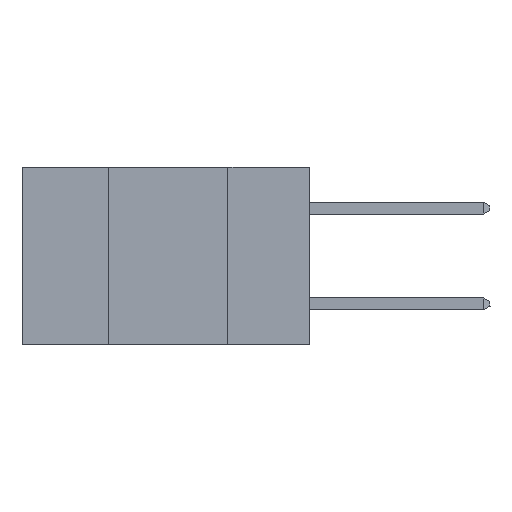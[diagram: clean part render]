
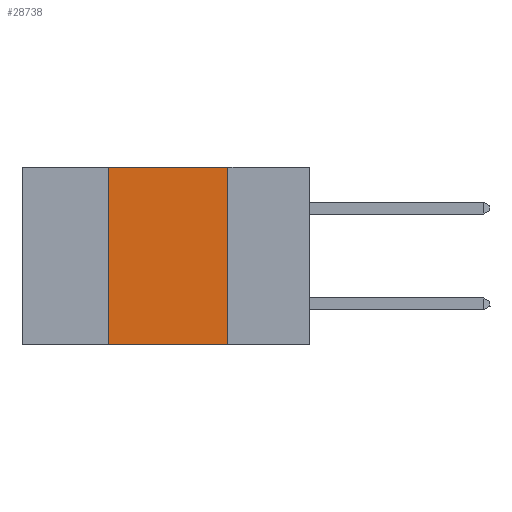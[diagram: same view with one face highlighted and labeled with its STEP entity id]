
A CAD part, left-side view. The second image highlights one B-rep face of the part: STEP entity #28738.
In plain terms, the highlighted planar face has unit normal (-1, 0, 0).
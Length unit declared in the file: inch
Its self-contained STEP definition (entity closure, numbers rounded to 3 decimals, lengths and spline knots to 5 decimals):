
#264 = PLANE ( 'NONE',  #30064 ) ;
#455 = CARTESIAN_POINT ( 'NONE',  ( 0., 0.42, 0. ) ) ;
#532 = VERTEX_POINT ( 'NONE', #7471 ) ;
#3584 = ORIENTED_EDGE ( 'NONE', *, *, #12356, .T. ) ;
#3883 = VECTOR ( 'NONE', #11330, 39.37008 ) ;
#3884 = EDGE_CURVE ( 'NONE', #7763, #26362, #16132, .T. ) ;
#7471 = CARTESIAN_POINT ( 'NONE',  ( 0., 0.17, -0.37 ) ) ;
#7547 = VECTOR ( 'NONE', #19287, 39.37008 ) ;
#7763 = VERTEX_POINT ( 'NONE', #20365 ) ;
#9404 = VECTOR ( 'NONE', #25095, 39.37008 ) ;
#11330 = DIRECTION ( 'NONE',  ( 0., -1., 0. ) ) ;
#12356 = EDGE_CURVE ( 'NONE', #7763, #532, #16015, .T. ) ;
#13783 = VERTEX_POINT ( 'NONE', #23346 ) ;
#14371 = EDGE_CURVE ( 'NONE', #26362, #13783, #29298, .T. ) ;
#16015 = LINE ( 'NONE', #26833, #3883 ) ;
#16132 = LINE ( 'NONE', #455, #20914 ) ;
#16338 = EDGE_LOOP ( 'NONE', ( #22075, #16587, #23740, #3584 ) ) ;
#16587 = ORIENTED_EDGE ( 'NONE', *, *, #14371, .F. ) ;
#18638 = DIRECTION ( 'NONE',  ( 0., 0., 1. ) ) ;
#19287 = DIRECTION ( 'NONE',  ( 0., -1., 0. ) ) ;
#19853 = CARTESIAN_POINT ( 'NONE',  ( 0., 0.42, 0. ) ) ;
#20365 = CARTESIAN_POINT ( 'NONE',  ( 0., 0.42, -0.37 ) ) ;
#20914 = VECTOR ( 'NONE', #18638, 39.37008 ) ;
#22075 = ORIENTED_EDGE ( 'NONE', *, *, #31052, .F. ) ;
#22120 = CARTESIAN_POINT ( 'NONE',  ( 0., 0.17, 0. ) ) ;
#22927 = DIRECTION ( 'NONE',  ( 0., 0., -1. ) ) ;
#23346 = CARTESIAN_POINT ( 'NONE',  ( 0., 0.17, 0. ) ) ;
#23740 = ORIENTED_EDGE ( 'NONE', *, *, #3884, .F. ) ;
#25095 = DIRECTION ( 'NONE',  ( 0., 0., -1. ) ) ;
#25277 = DIRECTION ( 'NONE',  ( 1., 0., 0. ) ) ;
#26362 = VERTEX_POINT ( 'NONE', #19853 ) ;
#26481 = CARTESIAN_POINT ( 'NONE',  ( 0., 0.6, 0. ) ) ;
#26833 = CARTESIAN_POINT ( 'NONE',  ( 0., 0.6, -0.37 ) ) ;
#28738 = ADVANCED_FACE ( 'NONE', ( #30428 ), #264, .F. ) ;
#29298 = LINE ( 'NONE', #26481, #7547 ) ;
#30064 = AXIS2_PLACEMENT_3D ( 'NONE', #30114, #25277, #22927 ) ;
#30114 = CARTESIAN_POINT ( 'NONE',  ( 0., 0.6, 0. ) ) ;
#30272 = LINE ( 'NONE', #22120, #9404 ) ;
#30428 = FACE_OUTER_BOUND ( 'NONE', #16338, .T. ) ;
#31052 = EDGE_CURVE ( 'NONE', #13783, #532, #30272, .T. ) ;
